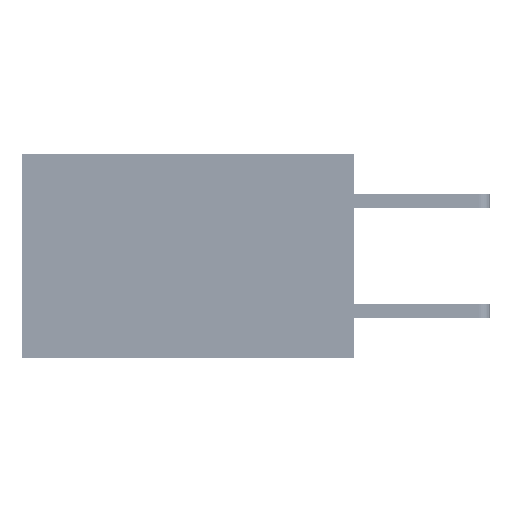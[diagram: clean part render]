
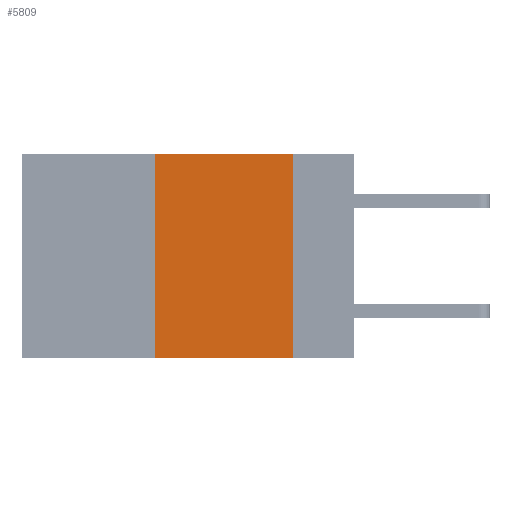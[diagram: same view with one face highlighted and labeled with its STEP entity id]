
A CAD part, left-side view. The second image highlights one B-rep face of the part: STEP entity #5809.
In plain terms, the highlighted planar face has unit normal (-1, 0, 0).
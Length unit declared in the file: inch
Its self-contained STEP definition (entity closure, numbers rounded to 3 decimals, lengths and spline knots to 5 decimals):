
#2546 = DIRECTION ( 'NONE',  ( 0., 0., -1. ) ) ;
#3436 = EDGE_CURVE ( 'NONE', #10980, #27971, #18951, .T. ) ;
#3986 = CARTESIAN_POINT ( 'NONE',  ( 0., 0.36, -0.37 ) ) ;
#4880 = EDGE_CURVE ( 'NONE', #30635, #40938, #16893, .T. ) ;
#5563 = LINE ( 'NONE', #5681, #30065 ) ;
#5681 = CARTESIAN_POINT ( 'NONE',  ( 0., 0.11, 0. ) ) ;
#5809 = ADVANCED_FACE ( 'NONE', ( #28943 ), #13151, .F. ) ;
#8760 = EDGE_CURVE ( 'NONE', #27971, #40938, #5563, .T. ) ;
#10655 = VECTOR ( 'NONE', #24427, 39.37008 ) ;
#10980 = VERTEX_POINT ( 'NONE', #11985 ) ;
#11985 = CARTESIAN_POINT ( 'NONE',  ( 0., 0.36, 0. ) ) ;
#13151 = PLANE ( 'NONE',  #33050 ) ;
#14560 = ORIENTED_EDGE ( 'NONE', *, *, #8760, .F. ) ;
#15951 = CARTESIAN_POINT ( 'NONE',  ( 0., 0.11, 0. ) ) ;
#16014 = CARTESIAN_POINT ( 'NONE',  ( 0., 0.6, -0.37 ) ) ;
#16510 = DIRECTION ( 'NONE',  ( 0., -1., 0. ) ) ;
#16893 = LINE ( 'NONE', #16014, #40933 ) ;
#18951 = LINE ( 'NONE', #39025, #39474 ) ;
#20120 = CARTESIAN_POINT ( 'NONE',  ( 0., 0.6, 0. ) ) ;
#21312 = DIRECTION ( 'NONE',  ( 1., 0., 0. ) ) ;
#23045 = ORIENTED_EDGE ( 'NONE', *, *, #4880, .T. ) ;
#24427 = DIRECTION ( 'NONE',  ( 0., 0., 1. ) ) ;
#25535 = EDGE_LOOP ( 'NONE', ( #14560, #27531, #38831, #23045 ) ) ;
#27531 = ORIENTED_EDGE ( 'NONE', *, *, #3436, .F. ) ;
#27670 = LINE ( 'NONE', #30684, #10655 ) ;
#27791 = CARTESIAN_POINT ( 'NONE',  ( 0., 0.11, -0.37 ) ) ;
#27971 = VERTEX_POINT ( 'NONE', #15951 ) ;
#28943 = FACE_OUTER_BOUND ( 'NONE', #25535, .T. ) ;
#30065 = VECTOR ( 'NONE', #2546, 39.37008 ) ;
#30635 = VERTEX_POINT ( 'NONE', #3986 ) ;
#30684 = CARTESIAN_POINT ( 'NONE',  ( 0., 0.36, 0. ) ) ;
#33050 = AXIS2_PLACEMENT_3D ( 'NONE', #20120, #21312, #40663 ) ;
#36671 = DIRECTION ( 'NONE',  ( 0., -1., 0. ) ) ;
#38831 = ORIENTED_EDGE ( 'NONE', *, *, #41371, .F. ) ;
#39025 = CARTESIAN_POINT ( 'NONE',  ( 0., 0.6, 0. ) ) ;
#39474 = VECTOR ( 'NONE', #16510, 39.37008 ) ;
#40663 = DIRECTION ( 'NONE',  ( 0., 0., -1. ) ) ;
#40933 = VECTOR ( 'NONE', #36671, 39.37008 ) ;
#40938 = VERTEX_POINT ( 'NONE', #27791 ) ;
#41371 = EDGE_CURVE ( 'NONE', #30635, #10980, #27670, .T. ) ;
